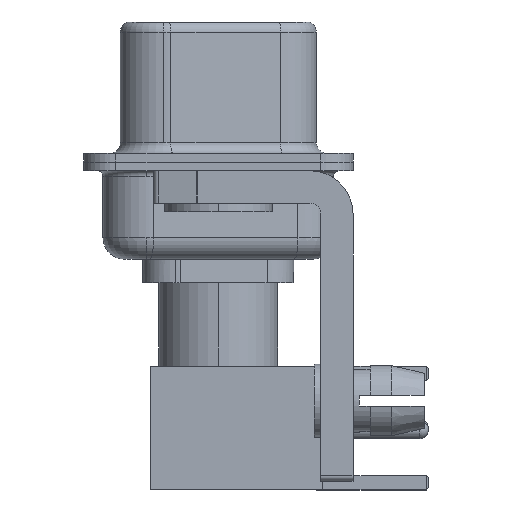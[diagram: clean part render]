
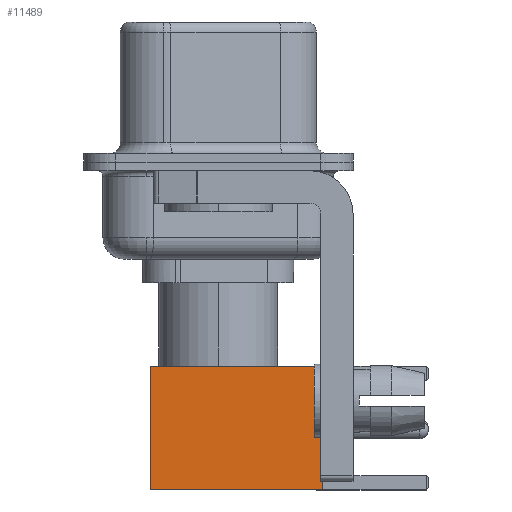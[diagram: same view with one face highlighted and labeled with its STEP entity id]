
A CAD part, left-side view. The second image highlights one B-rep face of the part: STEP entity #11489.
In plain terms, the highlighted face is planar.
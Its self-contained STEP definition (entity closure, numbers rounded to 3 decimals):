
#520 = VECTOR ( 'NONE', #2736, 1000. ) ;
#1666 = CARTESIAN_POINT ( 'NONE',  ( -2.875, 2.875, 0. ) ) ;
#1862 = FACE_OUTER_BOUND ( 'NONE', #21407, .T. ) ;
#2736 = DIRECTION ( 'NONE',  ( -1., 0., 0. ) ) ;
#2943 = VECTOR ( 'NONE', #12748, 1000. ) ;
#3402 = VERTEX_POINT ( 'NONE', #8138 ) ;
#5013 = ORIENTED_EDGE ( 'NONE', *, *, #8325, .F. ) ;
#5225 = VECTOR ( 'NONE', #18776, 1000. ) ;
#5520 = DIRECTION ( 'NONE',  ( 0., 0., 1. ) ) ;
#6812 = LINE ( 'NONE', #13557, #5225 ) ;
#6889 = VERTEX_POINT ( 'NONE', #10332 ) ;
#7927 = LINE ( 'NONE', #19794, #520 ) ;
#8064 = VERTEX_POINT ( 'NONE', #19563 ) ;
#8138 = CARTESIAN_POINT ( 'NONE',  ( 2.875, 2.875, 8. ) ) ;
#8325 = EDGE_CURVE ( 'NONE', #6889, #16193, #6812, .T. ) ;
#8624 = CARTESIAN_POINT ( 'NONE',  ( 2.875, 2.875, 0. ) ) ;
#8829 = EDGE_CURVE ( 'NONE', #3402, #8064, #12414, .T. ) ;
#8897 = CARTESIAN_POINT ( 'NONE',  ( 2.875, 2.875, 0. ) ) ;
#9108 = DIRECTION ( 'NONE',  ( 0., 0., -1. ) ) ;
#9543 = LINE ( 'NONE', #16287, #2943 ) ;
#10061 = ORIENTED_EDGE ( 'NONE', *, *, #19636, .F. ) ;
#10332 = CARTESIAN_POINT ( 'NONE',  ( -2.875, 2.875, 8. ) ) ;
#10816 = EDGE_CURVE ( 'NONE', #8064, #16193, #9543, .T. ) ;
#11420 = AXIS2_PLACEMENT_3D ( 'NONE', #8624, #15370, #5520 ) ;
#11489 = ADVANCED_FACE ( 'NONE', ( #1862 ), #17032, .T. ) ;
#12414 = LINE ( 'NONE', #8897, #17267 ) ;
#12748 = DIRECTION ( 'NONE',  ( -1., 0., 0. ) ) ;
#13557 = CARTESIAN_POINT ( 'NONE',  ( -2.875, 2.875, 0. ) ) ;
#15370 = DIRECTION ( 'NONE',  ( 0., 1., 0. ) ) ;
#16161 = ORIENTED_EDGE ( 'NONE', *, *, #8829, .T. ) ;
#16193 = VERTEX_POINT ( 'NONE', #1666 ) ;
#16287 = CARTESIAN_POINT ( 'NONE',  ( 0., 2.875, 0. ) ) ;
#17032 = PLANE ( 'NONE',  #11420 ) ;
#17267 = VECTOR ( 'NONE', #9108, 1000. ) ;
#18194 = ORIENTED_EDGE ( 'NONE', *, *, #10816, .T. ) ;
#18776 = DIRECTION ( 'NONE',  ( 0., 0., -1. ) ) ;
#19563 = CARTESIAN_POINT ( 'NONE',  ( 2.875, 2.875, 0. ) ) ;
#19636 = EDGE_CURVE ( 'NONE', #3402, #6889, #7927, .T. ) ;
#19794 = CARTESIAN_POINT ( 'NONE',  ( 0., 2.875, 8. ) ) ;
#21407 = EDGE_LOOP ( 'NONE', ( #16161, #18194, #5013, #10061 ) ) ;
